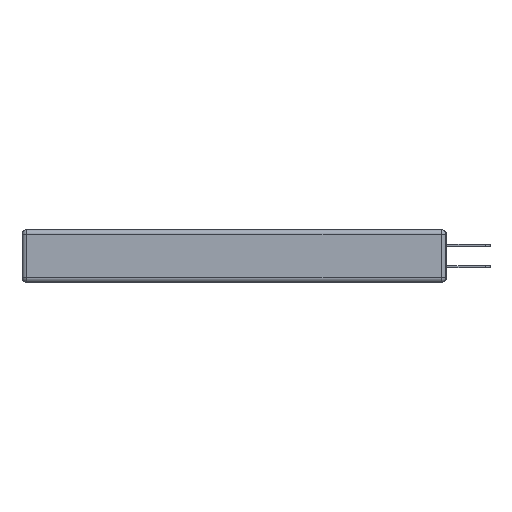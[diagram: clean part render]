
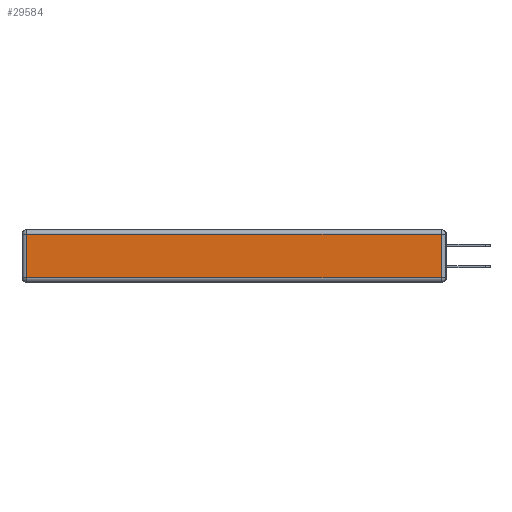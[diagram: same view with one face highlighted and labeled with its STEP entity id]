
A CAD part, left-side view. The second image highlights one B-rep face of the part: STEP entity #29584.
In plain terms, the highlighted planar face has unit normal (-1, 0, 0).
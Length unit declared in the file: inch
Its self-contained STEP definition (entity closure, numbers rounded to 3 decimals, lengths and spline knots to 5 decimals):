
#1319 = VERTEX_POINT ( 'NONE', #17919 ) ;
#1456 = PLANE ( 'NONE',  #23214 ) ;
#2001 = CARTESIAN_POINT ( 'NONE',  ( 0., 2.75, -0.03 ) ) ;
#3604 = ORIENTED_EDGE ( 'NONE', *, *, #22371, .T. ) ;
#3927 = CARTESIAN_POINT ( 'NONE',  ( 0., 0., -0.343 ) ) ;
#4517 = ORIENTED_EDGE ( 'NONE', *, *, #24266, .T. ) ;
#4766 = CARTESIAN_POINT ( 'NONE',  ( 0., 2.72, -0.03 ) ) ;
#6127 = EDGE_CURVE ( 'NONE', #1319, #14432, #9950, .T. ) ;
#7177 = ORIENTED_EDGE ( 'NONE', *, *, #16973, .T. ) ;
#7335 = CARTESIAN_POINT ( 'NONE',  ( 0., 0., -0.313 ) ) ;
#7967 = VERTEX_POINT ( 'NONE', #4766 ) ;
#8307 = VECTOR ( 'NONE', #12337, 39.37008 ) ;
#8552 = LINE ( 'NONE', #2001, #28202 ) ;
#8966 = DIRECTION ( 'NONE',  ( -1., 0., 0. ) ) ;
#9734 = FACE_OUTER_BOUND ( 'NONE', #15542, .T. ) ;
#9950 = LINE ( 'NONE', #27548, #12252 ) ;
#10008 = DIRECTION ( 'NONE',  ( 0., 0., 1. ) ) ;
#11478 = DIRECTION ( 'NONE',  ( 0., 0., 1. ) ) ;
#11694 = DIRECTION ( 'NONE',  ( 0., 1., 0. ) ) ;
#12252 = VECTOR ( 'NONE', #10008, 39.37008 ) ;
#12337 = DIRECTION ( 'NONE',  ( 0., -1., 0. ) ) ;
#12819 = VERTEX_POINT ( 'NONE', #18750 ) ;
#13065 = ORIENTED_EDGE ( 'NONE', *, *, #6127, .T. ) ;
#14432 = VERTEX_POINT ( 'NONE', #25943 ) ;
#15542 = EDGE_LOOP ( 'NONE', ( #7177, #13065, #3604, #4517 ) ) ;
#15700 = DIRECTION ( 'NONE',  ( 0., 0., -1. ) ) ;
#16973 = EDGE_CURVE ( 'NONE', #12819, #1319, #25678, .T. ) ;
#17919 = CARTESIAN_POINT ( 'NONE',  ( 0., 0.03, -0.313 ) ) ;
#18373 = CARTESIAN_POINT ( 'NONE',  ( 0., 2.72, -0.343 ) ) ;
#18519 = LINE ( 'NONE', #18373, #30855 ) ;
#18750 = CARTESIAN_POINT ( 'NONE',  ( 0., 2.72, -0.313 ) ) ;
#22371 = EDGE_CURVE ( 'NONE', #14432, #7967, #8552, .T. ) ;
#23214 = AXIS2_PLACEMENT_3D ( 'NONE', #3927, #8966, #11478 ) ;
#24266 = EDGE_CURVE ( 'NONE', #7967, #12819, #18519, .T. ) ;
#25678 = LINE ( 'NONE', #7335, #8307 ) ;
#25943 = CARTESIAN_POINT ( 'NONE',  ( 0., 0.03, -0.03 ) ) ;
#27548 = CARTESIAN_POINT ( 'NONE',  ( 0., 0.03, -0.343 ) ) ;
#28202 = VECTOR ( 'NONE', #11694, 39.37008 ) ;
#29584 = ADVANCED_FACE ( 'NONE', ( #9734 ), #1456, .T. ) ;
#30855 = VECTOR ( 'NONE', #15700, 39.37008 ) ;
